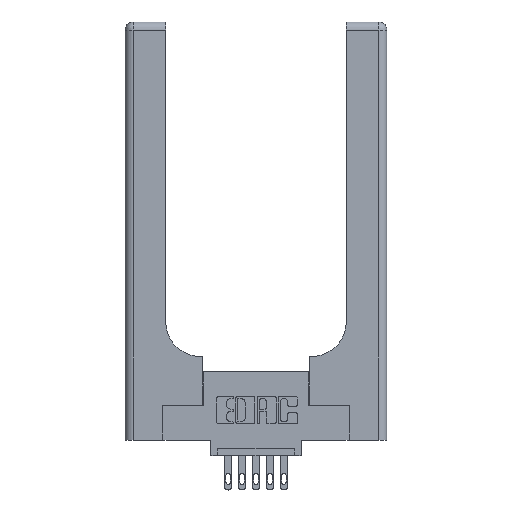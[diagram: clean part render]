
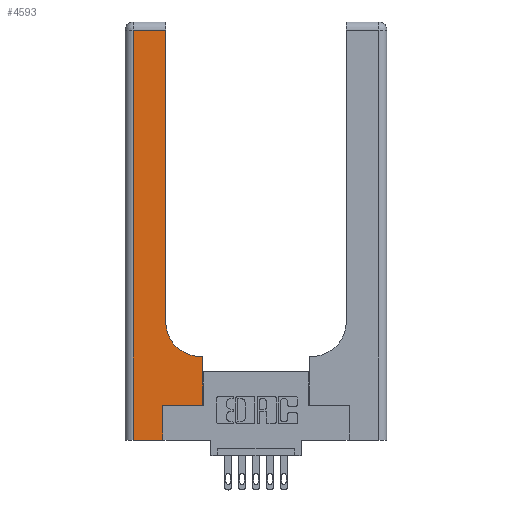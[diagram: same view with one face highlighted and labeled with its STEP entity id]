
A CAD part, top view. The second image highlights one B-rep face of the part: STEP entity #4593.
In plain terms, the highlighted planar face has unit normal (0, 0, 1).
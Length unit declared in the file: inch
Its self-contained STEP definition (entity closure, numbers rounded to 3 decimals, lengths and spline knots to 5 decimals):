
#12 = VERTEX_POINT ( 'NONE', #3506 ) ;
#644 = ORIENTED_EDGE ( 'NONE', *, *, #7805, .T. ) ;
#764 = CARTESIAN_POINT ( 'NONE',  ( 0.2915, 2.94, 0.37 ) ) ;
#1450 = DIRECTION ( 'NONE',  ( 1., 0., 0. ) ) ;
#1591 = CARTESIAN_POINT ( 'NONE',  ( 0.2915, 3., 0.37 ) ) ;
#1772 = ORIENTED_EDGE ( 'NONE', *, *, #9347, .T. ) ;
#2370 = LINE ( 'NONE', #4759, #4538 ) ;
#2375 = ORIENTED_EDGE ( 'NONE', *, *, #9673, .T. ) ;
#2399 = EDGE_CURVE ( 'NONE', #7855, #12, #3476, .T. ) ;
#2798 = LINE ( 'NONE', #6107, #4156 ) ;
#3476 = LINE ( 'NONE', #13628, #13112 ) ;
#3506 = CARTESIAN_POINT ( 'NONE',  ( 0.269, 0., 0.37 ) ) ;
#3535 = ORIENTED_EDGE ( 'NONE', *, *, #8787, .T. ) ;
#3815 = CARTESIAN_POINT ( 'NONE',  ( 0., 3., 0.37 ) ) ;
#3846 = ORIENTED_EDGE ( 'NONE', *, *, #9570, .T. ) ;
#3936 = DIRECTION ( 'NONE',  ( 1., 0., 0. ) ) ;
#3988 = ORIENTED_EDGE ( 'NONE', *, *, #2399, .T. ) ;
#4156 = VECTOR ( 'NONE', #7301, 39.37008 ) ;
#4386 = VERTEX_POINT ( 'NONE', #9797 ) ;
#4538 = VECTOR ( 'NONE', #9223, 39.37008 ) ;
#4593 = ADVANCED_FACE ( 'NONE', ( #11430 ), #6070, .F. ) ;
#4759 = CARTESIAN_POINT ( 'NONE',  ( 0., 2.94, 0.37 ) ) ;
#4817 = CARTESIAN_POINT ( 'NONE',  ( 0.2915, 0.85, 0.37 ) ) ;
#4909 = EDGE_LOOP ( 'NONE', ( #10564, #12126, #3846, #3988, #2375, #1772, #644, #7582, #3535 ) ) ;
#4952 = CARTESIAN_POINT ( 'NONE',  ( 0.06, 3., 0.37 ) ) ;
#4954 = DIRECTION ( 'NONE',  ( -1., 0., 0. ) ) ;
#4960 = CARTESIAN_POINT ( 'NONE',  ( 0.2915, 0.6, 0.37 ) ) ;
#4976 = LINE ( 'NONE', #1591, #6316 ) ;
#5063 = DIRECTION ( 'NONE',  ( -1., 0., 0. ) ) ;
#5316 = AXIS2_PLACEMENT_3D ( 'NONE', #10861, #6799, #1450 ) ;
#5579 = CARTESIAN_POINT ( 'NONE',  ( 0.06, 0., 0.37 ) ) ;
#5659 = DIRECTION ( 'NONE',  ( 0., 1., 0. ) ) ;
#5667 = VECTOR ( 'NONE', #8899, 39.37008 ) ;
#5701 = CARTESIAN_POINT ( 'NONE',  ( 0.269, 0.25, 0.37 ) ) ;
#6070 = PLANE ( 'NONE',  #13733 ) ;
#6085 = CARTESIAN_POINT ( 'NONE',  ( 0.06, 2.94, 0.37 ) ) ;
#6107 = CARTESIAN_POINT ( 'NONE',  ( 0.269, 0., 0.37 ) ) ;
#6316 = VECTOR ( 'NONE', #6803, 39.37008 ) ;
#6387 = VERTEX_POINT ( 'NONE', #9610 ) ;
#6768 = LINE ( 'NONE', #4960, #9979 ) ;
#6799 = DIRECTION ( 'NONE',  ( 0., 0., -1. ) ) ;
#6803 = DIRECTION ( 'NONE',  ( 0., 1., 0. ) ) ;
#7301 = DIRECTION ( 'NONE',  ( 0., 1., 0. ) ) ;
#7505 = VECTOR ( 'NONE', #10346, 39.37008 ) ;
#7582 = ORIENTED_EDGE ( 'NONE', *, *, #13686, .T. ) ;
#7774 = CARTESIAN_POINT ( 'NONE',  ( 0.269, 0.25, 0.37 ) ) ;
#7805 = EDGE_CURVE ( 'NONE', #4386, #6387, #11451, .T. ) ;
#7855 = VERTEX_POINT ( 'NONE', #5579 ) ;
#7920 = VERTEX_POINT ( 'NONE', #4817 ) ;
#8734 = VECTOR ( 'NONE', #5659, 39.37008 ) ;
#8787 = EDGE_CURVE ( 'NONE', #9788, #7920, #9879, .T. ) ;
#8812 = CARTESIAN_POINT ( 'NONE',  ( 0.5585, 0.25, 0.37 ) ) ;
#8831 = CARTESIAN_POINT ( 'NONE',  ( 0.5415, 0.6, 0.37 ) ) ;
#8899 = DIRECTION ( 'NONE',  ( 1., 0., 0. ) ) ;
#9223 = DIRECTION ( 'NONE',  ( -1., 0., 0. ) ) ;
#9347 = EDGE_CURVE ( 'NONE', #12353, #4386, #11571, .T. ) ;
#9570 = EDGE_CURVE ( 'NONE', #10338, #7855, #9860, .T. ) ;
#9610 = CARTESIAN_POINT ( 'NONE',  ( 0.5585, 0.6, 0.37 ) ) ;
#9673 = EDGE_CURVE ( 'NONE', #12, #12353, #2798, .T. ) ;
#9788 = VERTEX_POINT ( 'NONE', #8831 ) ;
#9797 = CARTESIAN_POINT ( 'NONE',  ( 0.5585, 0.25, 0.37 ) ) ;
#9860 = LINE ( 'NONE', #4952, #7505 ) ;
#9879 = CIRCLE ( 'NONE', #5316, 0.25 ) ;
#9969 = EDGE_CURVE ( 'NONE', #7920, #12154, #4976, .T. ) ;
#9979 = VECTOR ( 'NONE', #5063, 39.37008 ) ;
#10338 = VERTEX_POINT ( 'NONE', #6085 ) ;
#10346 = DIRECTION ( 'NONE',  ( 0., -1., 0. ) ) ;
#10564 = ORIENTED_EDGE ( 'NONE', *, *, #9969, .T. ) ;
#10832 = EDGE_CURVE ( 'NONE', #12154, #10338, #2370, .T. ) ;
#10861 = CARTESIAN_POINT ( 'NONE',  ( 0.5415, 0.85, 0.37 ) ) ;
#11430 = FACE_OUTER_BOUND ( 'NONE', #4909, .T. ) ;
#11451 = LINE ( 'NONE', #8812, #8734 ) ;
#11571 = LINE ( 'NONE', #5701, #5667 ) ;
#12126 = ORIENTED_EDGE ( 'NONE', *, *, #10832, .T. ) ;
#12154 = VERTEX_POINT ( 'NONE', #764 ) ;
#12353 = VERTEX_POINT ( 'NONE', #7774 ) ;
#13112 = VECTOR ( 'NONE', #3936, 39.37008 ) ;
#13568 = DIRECTION ( 'NONE',  ( 0., 0., -1. ) ) ;
#13628 = CARTESIAN_POINT ( 'NONE',  ( 0., 0., 0.37 ) ) ;
#13686 = EDGE_CURVE ( 'NONE', #6387, #9788, #6768, .T. ) ;
#13733 = AXIS2_PLACEMENT_3D ( 'NONE', #3815, #13568, #4954 ) ;
